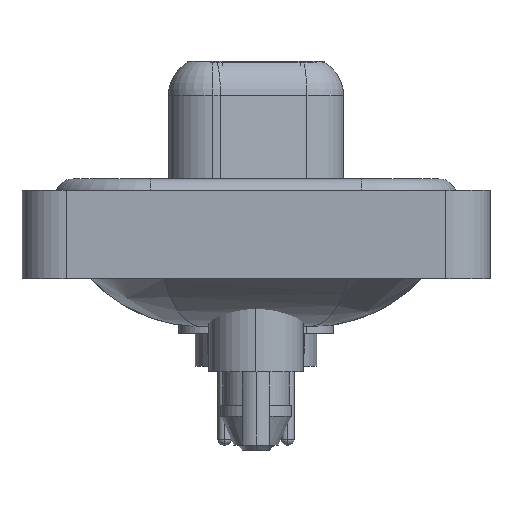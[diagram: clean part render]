
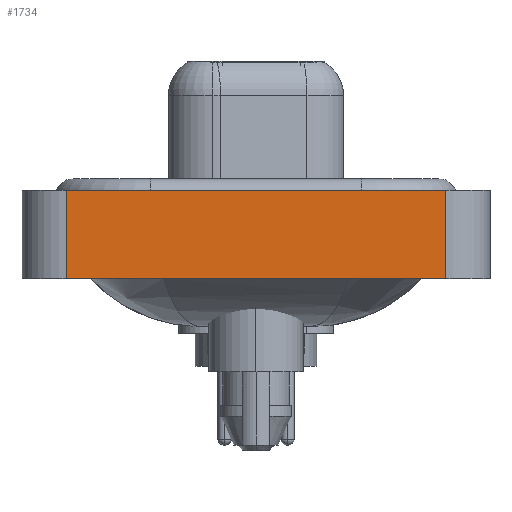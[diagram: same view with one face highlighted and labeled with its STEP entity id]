
A CAD part, left-side view. The second image highlights one B-rep face of the part: STEP entity #1734.
In plain terms, the highlighted planar face has unit normal (-1, 0, 0).
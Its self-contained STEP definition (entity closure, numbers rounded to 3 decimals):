
#426 = CARTESIAN_POINT ( 'NONE',  ( -7.3, -8.55, -3.6 ) ) ;
#602 = VERTEX_POINT ( 'NONE', #3903 ) ;
#729 = DIRECTION ( 'NONE',  ( 0., -1., 0. ) ) ;
#909 = EDGE_CURVE ( 'NONE', #4304, #22958, #7957, .T. ) ;
#1635 = CARTESIAN_POINT ( 'NONE',  ( -7.3, -8.55, 0.4 ) ) ;
#1734 = ADVANCED_FACE ( 'NONE', ( #2181 ), #5790, .T. ) ;
#1737 = ORIENTED_EDGE ( 'NONE', *, *, #7895, .T. ) ;
#1885 = DIRECTION ( 'NONE',  ( 0., 0., 1. ) ) ;
#2014 = CARTESIAN_POINT ( 'NONE',  ( -7.3, 8.55, -3.6 ) ) ;
#2181 = FACE_OUTER_BOUND ( 'NONE', #14037, .T. ) ;
#2364 = LINE ( 'NONE', #4223, #6407 ) ;
#3903 = CARTESIAN_POINT ( 'NONE',  ( -7.3, 8.55, -3.6 ) ) ;
#3998 = CARTESIAN_POINT ( 'NONE',  ( -7.3, -8.55, -3.6 ) ) ;
#4139 = AXIS2_PLACEMENT_3D ( 'NONE', #426, #7541, #14660 ) ;
#4223 = CARTESIAN_POINT ( 'NONE',  ( -7.3, -8.55, -3.6 ) ) ;
#4304 = VERTEX_POINT ( 'NONE', #12709 ) ;
#5216 = CARTESIAN_POINT ( 'NONE',  ( -7.3, -8.55, -3.6 ) ) ;
#5749 = LINE ( 'NONE', #3998, #18281 ) ;
#5790 = PLANE ( 'NONE',  #4139 ) ;
#6407 = VECTOR ( 'NONE', #16448, 1000. ) ;
#7541 = DIRECTION ( 'NONE',  ( -1., 0., 0. ) ) ;
#7866 = EDGE_CURVE ( 'NONE', #17159, #22958, #2364, .T. ) ;
#7895 = EDGE_CURVE ( 'NONE', #602, #17159, #5749, .T. ) ;
#7957 = LINE ( 'NONE', #16568, #13759 ) ;
#9012 = LINE ( 'NONE', #2014, #14237 ) ;
#9338 = EDGE_CURVE ( 'NONE', #602, #4304, #9012, .T. ) ;
#12709 = CARTESIAN_POINT ( 'NONE',  ( -7.3, 8.55, 0.4 ) ) ;
#12969 = DIRECTION ( 'NONE',  ( 0., -1., 0. ) ) ;
#13759 = VECTOR ( 'NONE', #729, 1000. ) ;
#14037 = EDGE_LOOP ( 'NONE', ( #16006, #16411, #14061, #1737 ) ) ;
#14061 = ORIENTED_EDGE ( 'NONE', *, *, #9338, .F. ) ;
#14237 = VECTOR ( 'NONE', #1885, 1000. ) ;
#14660 = DIRECTION ( 'NONE',  ( 0., 0., 1. ) ) ;
#16006 = ORIENTED_EDGE ( 'NONE', *, *, #7866, .T. ) ;
#16411 = ORIENTED_EDGE ( 'NONE', *, *, #909, .F. ) ;
#16448 = DIRECTION ( 'NONE',  ( 0., 0., 1. ) ) ;
#16568 = CARTESIAN_POINT ( 'NONE',  ( -7.3, -8.55, 0.4 ) ) ;
#17159 = VERTEX_POINT ( 'NONE', #5216 ) ;
#18281 = VECTOR ( 'NONE', #12969, 1000. ) ;
#22958 = VERTEX_POINT ( 'NONE', #1635 ) ;
